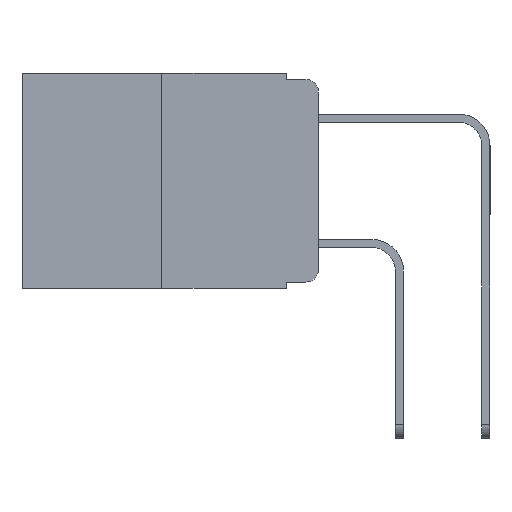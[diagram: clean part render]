
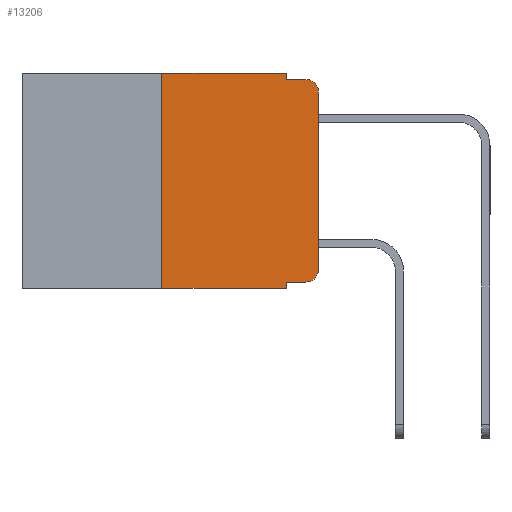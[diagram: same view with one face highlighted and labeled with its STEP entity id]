
A CAD part, left-side view. The second image highlights one B-rep face of the part: STEP entity #13206.
In plain terms, the highlighted planar face has unit normal (-1, 0, 0).
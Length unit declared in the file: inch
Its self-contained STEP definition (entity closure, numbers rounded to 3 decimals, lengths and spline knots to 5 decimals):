
#942 = CARTESIAN_POINT ( 'NONE',  ( 0., 0.02, -0.01 ) ) ;
#991 = AXIS2_PLACEMENT_3D ( 'NONE', #11645, #1296, #13333 ) ;
#1272 = EDGE_CURVE ( 'NONE', #2943, #9991, #15041, .T. ) ;
#1296 = DIRECTION ( 'NONE',  ( -1., 0., 0. ) ) ;
#1346 = EDGE_CURVE ( 'NONE', #18011, #19452, #13958, .T. ) ;
#1401 = VECTOR ( 'NONE', #8674, 39.37008 ) ;
#1628 = FACE_OUTER_BOUND ( 'NONE', #18936, .T. ) ;
#2710 = DIRECTION ( 'NONE',  ( -1., 0., 0. ) ) ;
#2716 = DIRECTION ( 'NONE',  ( 1., 0., 0. ) ) ;
#2943 = VERTEX_POINT ( 'NONE', #17079 ) ;
#2998 = CARTESIAN_POINT ( 'NONE',  ( 0., 0., -0.03 ) ) ;
#3052 = CARTESIAN_POINT ( 'NONE',  ( 0., 0.051, -0.343 ) ) ;
#3126 = CARTESIAN_POINT ( 'NONE',  ( 0., 0.051, -0.333 ) ) ;
#3268 = ORIENTED_EDGE ( 'NONE', *, *, #6718, .F. ) ;
#3453 = VECTOR ( 'NONE', #19944, 39.37008 ) ;
#3589 = CARTESIAN_POINT ( 'NONE',  ( 0., 0.051, 0. ) ) ;
#4020 = ORIENTED_EDGE ( 'NONE', *, *, #13598, .F. ) ;
#4079 = ORIENTED_EDGE ( 'NONE', *, *, #7143, .T. ) ;
#5578 = EDGE_CURVE ( 'NONE', #9349, #21249, #15928, .T. ) ;
#5707 = DIRECTION ( 'NONE',  ( 0., 0., 1. ) ) ;
#5913 = LINE ( 'NONE', #21856, #19333 ) ;
#6019 = VECTOR ( 'NONE', #8156, 39.37008 ) ;
#6247 = CARTESIAN_POINT ( 'NONE',  ( 0., 0.051, -0.01 ) ) ;
#6418 = EDGE_CURVE ( 'NONE', #13377, #11041, #8472, .T. ) ;
#6718 = EDGE_CURVE ( 'NONE', #18011, #9991, #15108, .T. ) ;
#6941 = VECTOR ( 'NONE', #15765, 39.37008 ) ;
#7143 = EDGE_CURVE ( 'NONE', #19452, #18042, #18166, .T. ) ;
#8156 = DIRECTION ( 'NONE',  ( 0., -1., 0. ) ) ;
#8378 = ORIENTED_EDGE ( 'NONE', *, *, #1272, .T. ) ;
#8380 = EDGE_CURVE ( 'NONE', #9333, #11041, #14730, .T. ) ;
#8472 = LINE ( 'NONE', #6247, #21807 ) ;
#8674 = DIRECTION ( 'NONE',  ( 0., 0., -1. ) ) ;
#8934 = VECTOR ( 'NONE', #14519, 39.37008 ) ;
#9333 = VERTEX_POINT ( 'NONE', #2998 ) ;
#9349 = VERTEX_POINT ( 'NONE', #9878 ) ;
#9878 = CARTESIAN_POINT ( 'NONE',  ( 0., 0.25, 0. ) ) ;
#9932 = CARTESIAN_POINT ( 'NONE',  ( 0., 0.051, 0. ) ) ;
#9991 = VERTEX_POINT ( 'NONE', #3052 ) ;
#10081 = EDGE_CURVE ( 'NONE', #18042, #9333, #5913, .T. ) ;
#11041 = VERTEX_POINT ( 'NONE', #942 ) ;
#11645 = CARTESIAN_POINT ( 'NONE',  ( 0., 0.02, -0.313 ) ) ;
#11769 = CARTESIAN_POINT ( 'NONE',  ( 0., 0., -0.313 ) ) ;
#12233 = CARTESIAN_POINT ( 'NONE',  ( 0., 0.02, -0.333 ) ) ;
#12478 = AXIS2_PLACEMENT_3D ( 'NONE', #12994, #2716, #14694 ) ;
#12989 = CARTESIAN_POINT ( 'NONE',  ( 0., 0.02, -0.03 ) ) ;
#12994 = CARTESIAN_POINT ( 'NONE',  ( 0., 0.473, 0. ) ) ;
#13206 = ADVANCED_FACE ( 'NONE', ( #1628 ), #17968, .F. ) ;
#13333 = DIRECTION ( 'NONE',  ( 0., 0., -1. ) ) ;
#13377 = VERTEX_POINT ( 'NONE', #18472 ) ;
#13598 = EDGE_CURVE ( 'NONE', #2943, #9349, #16110, .T. ) ;
#13928 = ORIENTED_EDGE ( 'NONE', *, *, #8380, .T. ) ;
#13958 = LINE ( 'NONE', #21692, #8934 ) ;
#14519 = DIRECTION ( 'NONE',  ( 0., -1., 0. ) ) ;
#14659 = AXIS2_PLACEMENT_3D ( 'NONE', #12989, #2710, #14688 ) ;
#14688 = DIRECTION ( 'NONE',  ( 0., 0., -1. ) ) ;
#14694 = DIRECTION ( 'NONE',  ( 0., 0., -1. ) ) ;
#14730 = CIRCLE ( 'NONE', #14659, 0.02 ) ;
#15041 = LINE ( 'NONE', #19411, #6019 ) ;
#15108 = LINE ( 'NONE', #3589, #1401 ) ;
#15765 = DIRECTION ( 'NONE',  ( 0., -1., 0. ) ) ;
#15816 = ORIENTED_EDGE ( 'NONE', *, *, #1346, .T. ) ;
#15861 = CARTESIAN_POINT ( 'NONE',  ( 0., 0.25, 0. ) ) ;
#15928 = LINE ( 'NONE', #19018, #6941 ) ;
#16110 = LINE ( 'NONE', #15861, #20507 ) ;
#16330 = ORIENTED_EDGE ( 'NONE', *, *, #6418, .F. ) ;
#16572 = ORIENTED_EDGE ( 'NONE', *, *, #20347, .F. ) ;
#16908 = DIRECTION ( 'NONE',  ( 0., 0., 1. ) ) ;
#17079 = CARTESIAN_POINT ( 'NONE',  ( 0., 0.25, -0.343 ) ) ;
#17968 = PLANE ( 'NONE',  #12478 ) ;
#18011 = VERTEX_POINT ( 'NONE', #3126 ) ;
#18042 = VERTEX_POINT ( 'NONE', #11769 ) ;
#18166 = CIRCLE ( 'NONE', #991, 0.02 ) ;
#18472 = CARTESIAN_POINT ( 'NONE',  ( 0., 0.051, -0.01 ) ) ;
#18670 = ORIENTED_EDGE ( 'NONE', *, *, #5578, .F. ) ;
#18936 = EDGE_LOOP ( 'NONE', ( #21403, #13928, #16330, #16572, #18670, #4020, #8378, #3268, #15816, #4079 ) ) ;
#19018 = CARTESIAN_POINT ( 'NONE',  ( 0., 0.473, 0. ) ) ;
#19333 = VECTOR ( 'NONE', #16908, 39.37008 ) ;
#19411 = CARTESIAN_POINT ( 'NONE',  ( 0., 0.473, -0.343 ) ) ;
#19452 = VERTEX_POINT ( 'NONE', #12233 ) ;
#19685 = DIRECTION ( 'NONE',  ( 0., -1., 0. ) ) ;
#19944 = DIRECTION ( 'NONE',  ( 0., 0., -1. ) ) ;
#20347 = EDGE_CURVE ( 'NONE', #21249, #13377, #20887, .T. ) ;
#20507 = VECTOR ( 'NONE', #5707, 39.37008 ) ;
#20715 = CARTESIAN_POINT ( 'NONE',  ( 0., 0.051, 0. ) ) ;
#20887 = LINE ( 'NONE', #9932, #3453 ) ;
#21249 = VERTEX_POINT ( 'NONE', #20715 ) ;
#21403 = ORIENTED_EDGE ( 'NONE', *, *, #10081, .T. ) ;
#21692 = CARTESIAN_POINT ( 'NONE',  ( 0., 0.051, -0.333 ) ) ;
#21807 = VECTOR ( 'NONE', #19685, 39.37008 ) ;
#21856 = CARTESIAN_POINT ( 'NONE',  ( 0., 0., 0. ) ) ;
